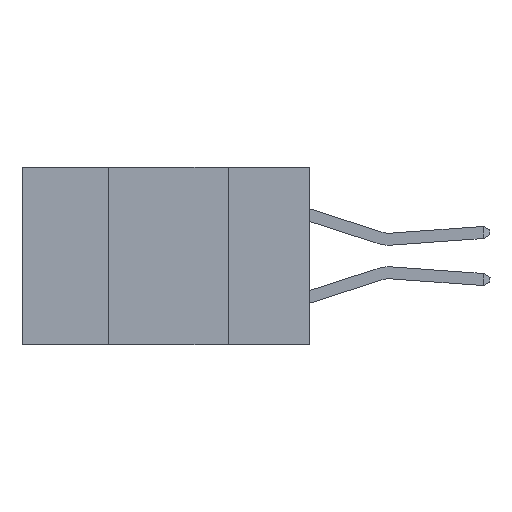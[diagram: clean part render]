
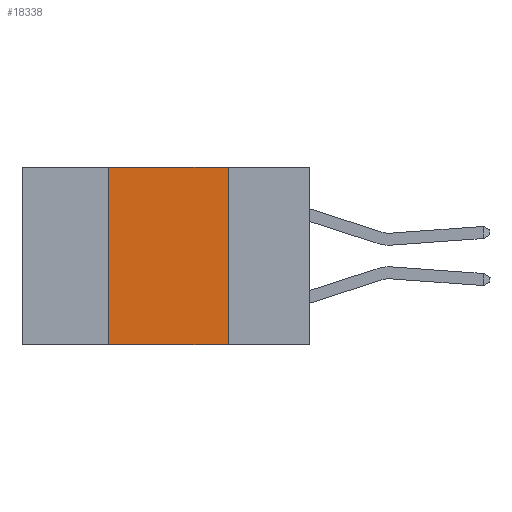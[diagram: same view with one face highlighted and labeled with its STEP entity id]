
A CAD part, left-side view. The second image highlights one B-rep face of the part: STEP entity #18338.
In plain terms, the highlighted planar face has unit normal (-1, 0, 0).
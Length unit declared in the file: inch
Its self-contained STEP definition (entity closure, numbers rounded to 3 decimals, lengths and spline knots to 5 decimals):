
#1230 = VERTEX_POINT ( 'NONE', #17700 ) ;
#1801 = CARTESIAN_POINT ( 'NONE',  ( 0., 0.42, -0.37 ) ) ;
#1868 = PLANE ( 'NONE',  #20155 ) ;
#2103 = LINE ( 'NONE', #6086, #10440 ) ;
#2694 = VERTEX_POINT ( 'NONE', #18099 ) ;
#2834 = ORIENTED_EDGE ( 'NONE', *, *, #14097, .F. ) ;
#3436 = DIRECTION ( 'NONE',  ( 0., 0., 1. ) ) ;
#3654 = DIRECTION ( 'NONE',  ( 0., -1., 0. ) ) ;
#4071 = VECTOR ( 'NONE', #20720, 39.37008 ) ;
#4487 = FACE_OUTER_BOUND ( 'NONE', #20990, .T. ) ;
#4630 = VECTOR ( 'NONE', #3436, 39.37008 ) ;
#5103 = VERTEX_POINT ( 'NONE', #11518 ) ;
#6086 = CARTESIAN_POINT ( 'NONE',  ( 0., 0.6, -0.37 ) ) ;
#6158 = DIRECTION ( 'NONE',  ( 0., -1., 0. ) ) ;
#7477 = EDGE_CURVE ( 'NONE', #5103, #21141, #12918, .T. ) ;
#7657 = VECTOR ( 'NONE', #3654, 39.37008 ) ;
#7796 = ORIENTED_EDGE ( 'NONE', *, *, #9684, .F. ) ;
#9684 = EDGE_CURVE ( 'NONE', #2694, #5103, #13069, .T. ) ;
#10239 = DIRECTION ( 'NONE',  ( 0., 0., -1. ) ) ;
#10440 = VECTOR ( 'NONE', #6158, 39.37008 ) ;
#11518 = CARTESIAN_POINT ( 'NONE',  ( 0., 0.17, 0. ) ) ;
#11949 = CARTESIAN_POINT ( 'NONE',  ( 0., 0.6, 0. ) ) ;
#12918 = LINE ( 'NONE', #17517, #4071 ) ;
#13069 = LINE ( 'NONE', #11949, #7657 ) ;
#14097 = EDGE_CURVE ( 'NONE', #1230, #2694, #17796, .T. ) ;
#14258 = ORIENTED_EDGE ( 'NONE', *, *, #19538, .T. ) ;
#17517 = CARTESIAN_POINT ( 'NONE',  ( 0., 0.17, -0.37 ) ) ;
#17700 = CARTESIAN_POINT ( 'NONE',  ( 0., 0.42, -0.37 ) ) ;
#17796 = LINE ( 'NONE', #1801, #4630 ) ;
#18099 = CARTESIAN_POINT ( 'NONE',  ( 0., 0.42, 0. ) ) ;
#18113 = CARTESIAN_POINT ( 'NONE',  ( 0., 0.17, -0.37 ) ) ;
#18338 = ADVANCED_FACE ( 'NONE', ( #4487 ), #1868, .F. ) ;
#18400 = CARTESIAN_POINT ( 'NONE',  ( 0., 0.6, 0. ) ) ;
#19538 = EDGE_CURVE ( 'NONE', #1230, #21141, #2103, .T. ) ;
#19561 = ORIENTED_EDGE ( 'NONE', *, *, #7477, .F. ) ;
#20007 = DIRECTION ( 'NONE',  ( 1., 0., 0. ) ) ;
#20155 = AXIS2_PLACEMENT_3D ( 'NONE', #18400, #20007, #10239 ) ;
#20720 = DIRECTION ( 'NONE',  ( 0., 0., -1. ) ) ;
#20990 = EDGE_LOOP ( 'NONE', ( #19561, #7796, #2834, #14258 ) ) ;
#21141 = VERTEX_POINT ( 'NONE', #18113 ) ;
